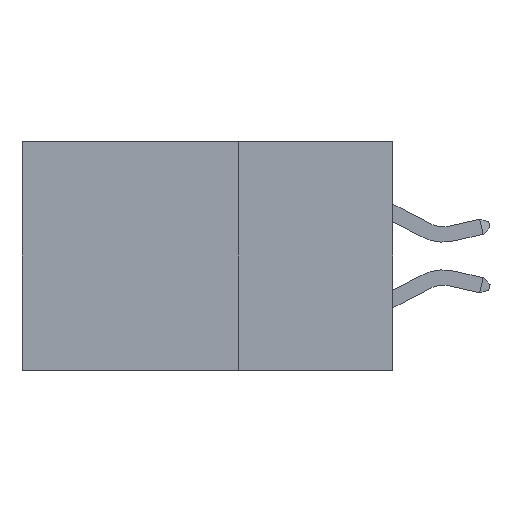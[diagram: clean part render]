
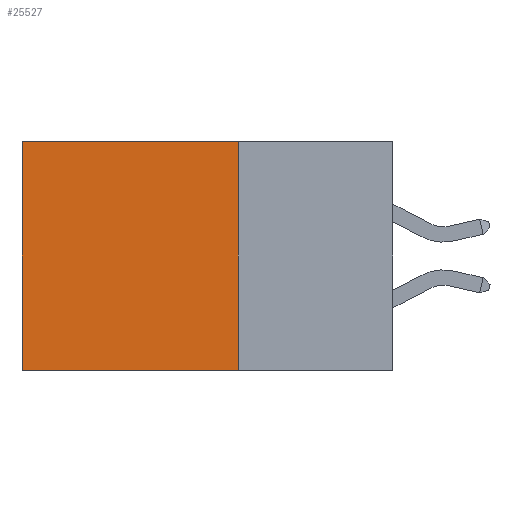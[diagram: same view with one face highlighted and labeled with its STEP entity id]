
A CAD part, left-side view. The second image highlights one B-rep face of the part: STEP entity #25527.
In plain terms, the highlighted planar face has unit normal (-1, 0, 0).
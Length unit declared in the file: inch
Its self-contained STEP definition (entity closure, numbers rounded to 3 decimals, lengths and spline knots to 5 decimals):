
#254 = EDGE_CURVE ( 'NONE', #26197, #4776, #20253, .T. ) ;
#736 = CARTESIAN_POINT ( 'NONE',  ( 0.2875, 0.25, 0. ) ) ;
#899 = EDGE_CURVE ( 'NONE', #9931, #11280, #4405, .T. ) ;
#1594 = CARTESIAN_POINT ( 'NONE',  ( 0.2875, 0.6, 0. ) ) ;
#2473 = DIRECTION ( 'NONE',  ( 0., 0., -1. ) ) ;
#3620 = DIRECTION ( 'NONE',  ( 0., 0., -1. ) ) ;
#4405 = LINE ( 'NONE', #24096, #14984 ) ;
#4615 = CARTESIAN_POINT ( 'NONE',  ( 0.2875, 0.25, 0. ) ) ;
#4776 = VERTEX_POINT ( 'NONE', #13717 ) ;
#5104 = LINE ( 'NONE', #6263, #26697 ) ;
#5183 = EDGE_CURVE ( 'NONE', #9931, #26197, #11145, .T. ) ;
#6263 = CARTESIAN_POINT ( 'NONE',  ( 0.2875, 0.6, 0. ) ) ;
#9254 = ORIENTED_EDGE ( 'NONE', *, *, #254, .F. ) ;
#9931 = VERTEX_POINT ( 'NONE', #736 ) ;
#10000 = EDGE_LOOP ( 'NONE', ( #26851, #9254, #26548, #13988 ) ) ;
#10504 = DIRECTION ( 'NONE',  ( 0., 0., -1. ) ) ;
#11145 = LINE ( 'NONE', #4615, #16769 ) ;
#11280 = VERTEX_POINT ( 'NONE', #1594 ) ;
#12059 = FACE_OUTER_BOUND ( 'NONE', #10000, .T. ) ;
#12068 = CARTESIAN_POINT ( 'NONE',  ( 0.2875, 0.25, 0. ) ) ;
#13717 = CARTESIAN_POINT ( 'NONE',  ( 0.2875, 0.6, -0.37 ) ) ;
#13988 = ORIENTED_EDGE ( 'NONE', *, *, #899, .T. ) ;
#14146 = CARTESIAN_POINT ( 'NONE',  ( 0.2875, 0.25, -0.37 ) ) ;
#14177 = PLANE ( 'NONE',  #25062 ) ;
#14984 = VECTOR ( 'NONE', #22054, 39.37008 ) ;
#16316 = DIRECTION ( 'NONE',  ( 1., 0., 0. ) ) ;
#16334 = CARTESIAN_POINT ( 'NONE',  ( 0.2875, 0.25, -0.37 ) ) ;
#16472 = DIRECTION ( 'NONE',  ( 0., 1., 0. ) ) ;
#16769 = VECTOR ( 'NONE', #2473, 39.37008 ) ;
#19620 = VECTOR ( 'NONE', #16472, 39.37008 ) ;
#20253 = LINE ( 'NONE', #16334, #19620 ) ;
#22054 = DIRECTION ( 'NONE',  ( 0., 1., 0. ) ) ;
#24096 = CARTESIAN_POINT ( 'NONE',  ( 0.2875, 0.25, 0. ) ) ;
#24465 = EDGE_CURVE ( 'NONE', #11280, #4776, #5104, .T. ) ;
#25062 = AXIS2_PLACEMENT_3D ( 'NONE', #12068, #16316, #3620 ) ;
#25527 = ADVANCED_FACE ( 'NONE', ( #12059 ), #14177, .F. ) ;
#26197 = VERTEX_POINT ( 'NONE', #14146 ) ;
#26548 = ORIENTED_EDGE ( 'NONE', *, *, #5183, .F. ) ;
#26697 = VECTOR ( 'NONE', #10504, 39.37008 ) ;
#26851 = ORIENTED_EDGE ( 'NONE', *, *, #24465, .T. ) ;
